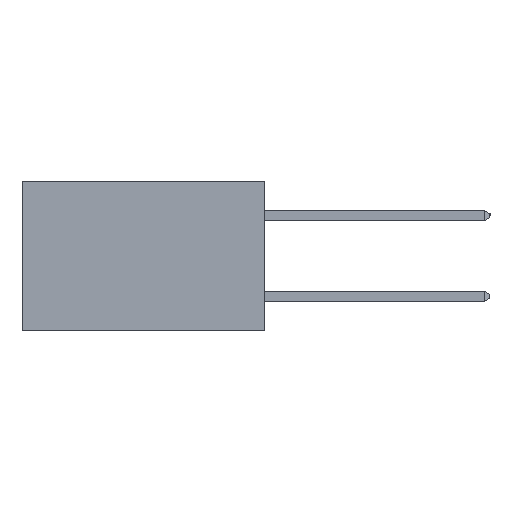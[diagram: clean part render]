
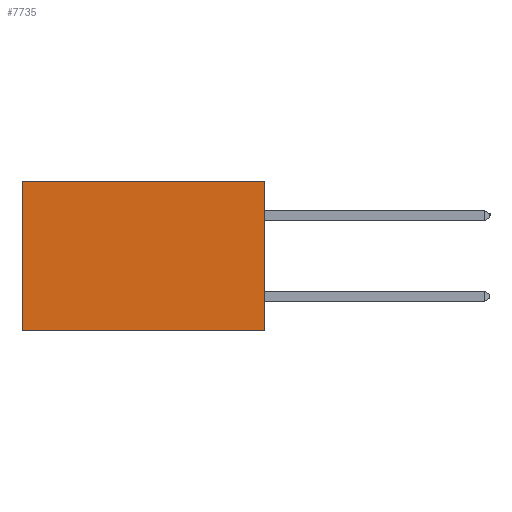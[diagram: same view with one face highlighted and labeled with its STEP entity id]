
A CAD part, left-side view. The second image highlights one B-rep face of the part: STEP entity #7735.
In plain terms, the highlighted planar face has unit normal (-1, 0, 0).
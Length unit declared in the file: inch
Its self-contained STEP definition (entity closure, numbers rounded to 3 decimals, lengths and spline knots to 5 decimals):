
#116 = ORIENTED_EDGE ( 'NONE', *, *, #17315, .T. ) ;
#1401 = PLANE ( 'NONE',  #12410 ) ;
#2300 = EDGE_CURVE ( 'NONE', #4822, #16266, #19536, .T. ) ;
#2987 = DIRECTION ( 'NONE',  ( 0., 0., -1. ) ) ;
#3336 = EDGE_LOOP ( 'NONE', ( #11813, #10947, #16365, #116 ) ) ;
#3360 = CARTESIAN_POINT ( 'NONE',  ( 0.2615, 0., 0. ) ) ;
#4479 = FACE_OUTER_BOUND ( 'NONE', #3336, .T. ) ;
#4822 = VERTEX_POINT ( 'NONE', #9822 ) ;
#5821 = CARTESIAN_POINT ( 'NONE',  ( 0.2615, 0., -0.37 ) ) ;
#6158 = VECTOR ( 'NONE', #8986, 39.37008 ) ;
#6649 = DIRECTION ( 'NONE',  ( 0., 1., 0. ) ) ;
#7165 = CARTESIAN_POINT ( 'NONE',  ( 0.2615, 0.6, -0.37 ) ) ;
#7508 = CARTESIAN_POINT ( 'NONE',  ( 0.2615, 0., -0.37 ) ) ;
#7735 = ADVANCED_FACE ( 'NONE', ( #4479 ), #1401, .F. ) ;
#8947 = DIRECTION ( 'NONE',  ( 1., 0., 0. ) ) ;
#8986 = DIRECTION ( 'NONE',  ( 0., 0., -1. ) ) ;
#9501 = CARTESIAN_POINT ( 'NONE',  ( 0.2615, 0., -0.37 ) ) ;
#9822 = CARTESIAN_POINT ( 'NONE',  ( 0.2615, 0.6, 0. ) ) ;
#10804 = LINE ( 'NONE', #3360, #15919 ) ;
#10947 = ORIENTED_EDGE ( 'NONE', *, *, #18208, .F. ) ;
#11813 = ORIENTED_EDGE ( 'NONE', *, *, #2300, .T. ) ;
#11854 = DIRECTION ( 'NONE',  ( 0., 1., 0. ) ) ;
#12178 = VERTEX_POINT ( 'NONE', #13442 ) ;
#12410 = AXIS2_PLACEMENT_3D ( 'NONE', #13492, #8947, #2987 ) ;
#13329 = LINE ( 'NONE', #7508, #6158 ) ;
#13442 = CARTESIAN_POINT ( 'NONE',  ( 0.2615, 0., 0. ) ) ;
#13492 = CARTESIAN_POINT ( 'NONE',  ( 0.2615, 0., -0.37 ) ) ;
#14786 = VECTOR ( 'NONE', #19249, 39.37008 ) ;
#15919 = VECTOR ( 'NONE', #6649, 39.37008 ) ;
#16048 = CARTESIAN_POINT ( 'NONE',  ( 0.2615, 0.6, -0.37 ) ) ;
#16163 = VERTEX_POINT ( 'NONE', #9501 ) ;
#16259 = VECTOR ( 'NONE', #11854, 39.37008 ) ;
#16266 = VERTEX_POINT ( 'NONE', #16048 ) ;
#16365 = ORIENTED_EDGE ( 'NONE', *, *, #18153, .F. ) ;
#17315 = EDGE_CURVE ( 'NONE', #12178, #4822, #10804, .T. ) ;
#18153 = EDGE_CURVE ( 'NONE', #12178, #16163, #13329, .T. ) ;
#18208 = EDGE_CURVE ( 'NONE', #16163, #16266, #19388, .T. ) ;
#19249 = DIRECTION ( 'NONE',  ( 0., 0., -1. ) ) ;
#19388 = LINE ( 'NONE', #5821, #16259 ) ;
#19536 = LINE ( 'NONE', #7165, #14786 ) ;
